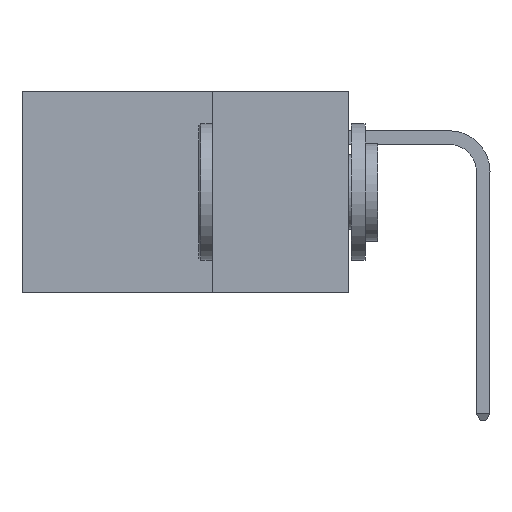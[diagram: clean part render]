
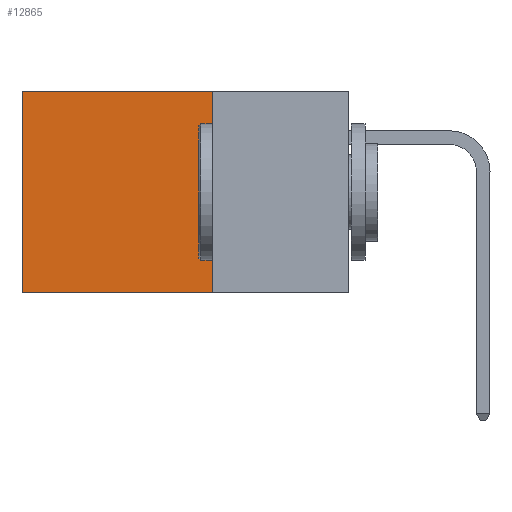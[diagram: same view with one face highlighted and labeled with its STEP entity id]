
A CAD part, left-side view. The second image highlights one B-rep face of the part: STEP entity #12865.
In plain terms, the highlighted planar face has unit normal (-1, 0, 0).
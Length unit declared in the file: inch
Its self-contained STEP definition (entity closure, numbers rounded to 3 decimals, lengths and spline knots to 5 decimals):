
#795 = LINE ( 'NONE', #3510, #15688 ) ;
#878 = EDGE_LOOP ( 'NONE', ( #3217, #15595, #8195, #15070 ) ) ;
#887 = FACE_OUTER_BOUND ( 'NONE', #878, .T. ) ;
#2708 = EDGE_CURVE ( 'NONE', #15751, #4495, #795, .T. ) ;
#2751 = CARTESIAN_POINT ( 'NONE',  ( 0.2875, 0.25, 0. ) ) ;
#3217 = ORIENTED_EDGE ( 'NONE', *, *, #22838, .T. ) ;
#3510 = CARTESIAN_POINT ( 'NONE',  ( 0.2875, 0.25, 0. ) ) ;
#3977 = PLANE ( 'NONE',  #7989 ) ;
#4108 = CARTESIAN_POINT ( 'NONE',  ( 0.2875, 0.25, -0.37 ) ) ;
#4211 = CARTESIAN_POINT ( 'NONE',  ( 0.2875, 0.25, 0. ) ) ;
#4495 = VERTEX_POINT ( 'NONE', #17182 ) ;
#4582 = VECTOR ( 'NONE', #14819, 39.37008 ) ;
#5469 = EDGE_CURVE ( 'NONE', #15751, #16881, #18179, .T. ) ;
#5847 = DIRECTION ( 'NONE',  ( 1., 0., 0. ) ) ;
#7002 = DIRECTION ( 'NONE',  ( 0., 0., -1. ) ) ;
#7989 = AXIS2_PLACEMENT_3D ( 'NONE', #16504, #5847, #18250 ) ;
#8195 = ORIENTED_EDGE ( 'NONE', *, *, #2708, .F. ) ;
#8779 = LINE ( 'NONE', #4108, #4582 ) ;
#10439 = VECTOR ( 'NONE', #14917, 39.37008 ) ;
#12595 = CARTESIAN_POINT ( 'NONE',  ( 0.2875, 0.6, 0. ) ) ;
#12672 = DIRECTION ( 'NONE',  ( 0., 0., -1. ) ) ;
#12865 = ADVANCED_FACE ( 'NONE', ( #887 ), #3977, .F. ) ;
#13426 = EDGE_CURVE ( 'NONE', #4495, #20948, #8779, .T. ) ;
#14819 = DIRECTION ( 'NONE',  ( 0., 1., 0. ) ) ;
#14917 = DIRECTION ( 'NONE',  ( 0., 1., 0. ) ) ;
#15070 = ORIENTED_EDGE ( 'NONE', *, *, #5469, .T. ) ;
#15595 = ORIENTED_EDGE ( 'NONE', *, *, #13426, .F. ) ;
#15688 = VECTOR ( 'NONE', #7002, 39.37008 ) ;
#15751 = VERTEX_POINT ( 'NONE', #2751 ) ;
#15848 = CARTESIAN_POINT ( 'NONE',  ( 0.2875, 0.6, 0. ) ) ;
#16034 = CARTESIAN_POINT ( 'NONE',  ( 0.2875, 0.6, -0.37 ) ) ;
#16504 = CARTESIAN_POINT ( 'NONE',  ( 0.2875, 0.25, 0. ) ) ;
#16881 = VERTEX_POINT ( 'NONE', #15848 ) ;
#17182 = CARTESIAN_POINT ( 'NONE',  ( 0.2875, 0.25, -0.37 ) ) ;
#18179 = LINE ( 'NONE', #4211, #10439 ) ;
#18250 = DIRECTION ( 'NONE',  ( 0., 0., -1. ) ) ;
#18722 = LINE ( 'NONE', #12595, #22268 ) ;
#20948 = VERTEX_POINT ( 'NONE', #16034 ) ;
#22268 = VECTOR ( 'NONE', #12672, 39.37008 ) ;
#22838 = EDGE_CURVE ( 'NONE', #16881, #20948, #18722, .T. ) ;
